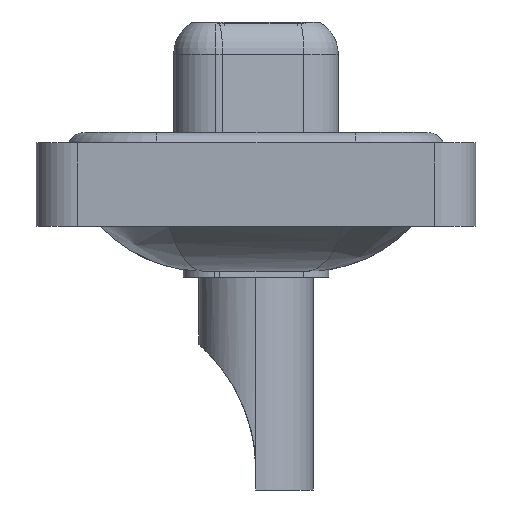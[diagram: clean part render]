
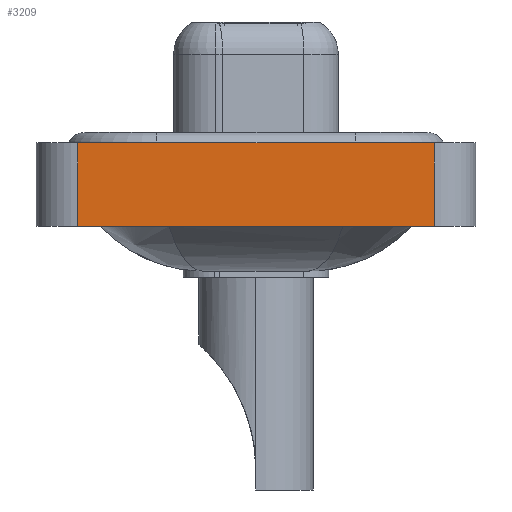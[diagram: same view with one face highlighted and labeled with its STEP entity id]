
A CAD part, left-side view. The second image highlights one B-rep face of the part: STEP entity #3209.
In plain terms, the highlighted planar face has unit normal (-1, 0, 0).
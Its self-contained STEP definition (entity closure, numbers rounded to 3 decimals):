
#382 = CARTESIAN_POINT ( 'NONE',  ( -7.3, 8.55, -3.6 ) ) ;
#970 = CARTESIAN_POINT ( 'NONE',  ( -7.3, -8.55, 0.4 ) ) ;
#980 = EDGE_LOOP ( 'NONE', ( #5593, #5950, #9039, #19794 ) ) ;
#1787 = LINE ( 'NONE', #3288, #10459 ) ;
#2199 = VECTOR ( 'NONE', #8401, 1000. ) ;
#2498 = VERTEX_POINT ( 'NONE', #4270 ) ;
#2527 = VERTEX_POINT ( 'NONE', #6459 ) ;
#2672 = CARTESIAN_POINT ( 'NONE',  ( -7.3, 8.55, -3.6 ) ) ;
#3209 = ADVANCED_FACE ( 'NONE', ( #13152 ), #8512, .T. ) ;
#3288 = CARTESIAN_POINT ( 'NONE',  ( -7.3, -8.55, -3.6 ) ) ;
#4270 = CARTESIAN_POINT ( 'NONE',  ( -7.3, 8.55, 0.4 ) ) ;
#5144 = CARTESIAN_POINT ( 'NONE',  ( -7.3, -8.55, -3.6 ) ) ;
#5252 = LINE ( 'NONE', #382, #2199 ) ;
#5593 = ORIENTED_EDGE ( 'NONE', *, *, #9282, .T. ) ;
#5741 = LINE ( 'NONE', #970, #7127 ) ;
#5950 = ORIENTED_EDGE ( 'NONE', *, *, #17312, .F. ) ;
#6038 = EDGE_CURVE ( 'NONE', #15311, #11414, #1787, .T. ) ;
#6459 = CARTESIAN_POINT ( 'NONE',  ( -7.3, -8.55, 0.4 ) ) ;
#6532 = DIRECTION ( 'NONE',  ( -1., 0., 0. ) ) ;
#7127 = VECTOR ( 'NONE', #7402, 1000. ) ;
#7380 = DIRECTION ( 'NONE',  ( 0., 0., 1. ) ) ;
#7402 = DIRECTION ( 'NONE',  ( 0., -1., 0. ) ) ;
#8401 = DIRECTION ( 'NONE',  ( 0., 0., 1. ) ) ;
#8512 = PLANE ( 'NONE',  #20442 ) ;
#9039 = ORIENTED_EDGE ( 'NONE', *, *, #11395, .F. ) ;
#9282 = EDGE_CURVE ( 'NONE', #11414, #2527, #10557, .T. ) ;
#10106 = DIRECTION ( 'NONE',  ( 0., 0., 1. ) ) ;
#10459 = VECTOR ( 'NONE', #14833, 1000. ) ;
#10557 = LINE ( 'NONE', #16963, #10884 ) ;
#10884 = VECTOR ( 'NONE', #7380, 1000. ) ;
#11395 = EDGE_CURVE ( 'NONE', #15311, #2498, #5252, .T. ) ;
#11414 = VERTEX_POINT ( 'NONE', #5144 ) ;
#13152 = FACE_OUTER_BOUND ( 'NONE', #980, .T. ) ;
#14722 = CARTESIAN_POINT ( 'NONE',  ( -7.3, -8.55, -3.6 ) ) ;
#14833 = DIRECTION ( 'NONE',  ( 0., -1., 0. ) ) ;
#15311 = VERTEX_POINT ( 'NONE', #2672 ) ;
#16963 = CARTESIAN_POINT ( 'NONE',  ( -7.3, -8.55, -3.6 ) ) ;
#17312 = EDGE_CURVE ( 'NONE', #2498, #2527, #5741, .T. ) ;
#19794 = ORIENTED_EDGE ( 'NONE', *, *, #6038, .T. ) ;
#20442 = AXIS2_PLACEMENT_3D ( 'NONE', #14722, #6532, #10106 ) ;
